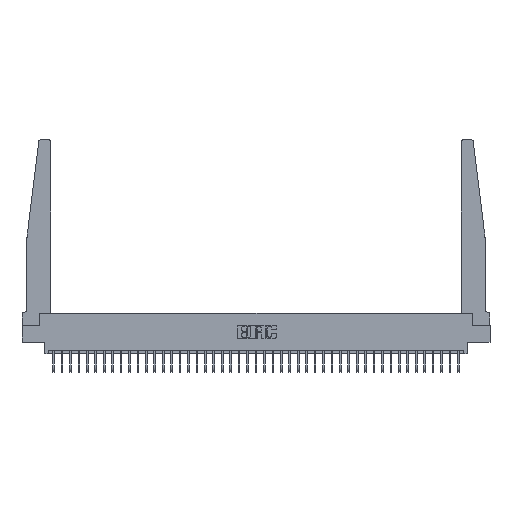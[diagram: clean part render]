
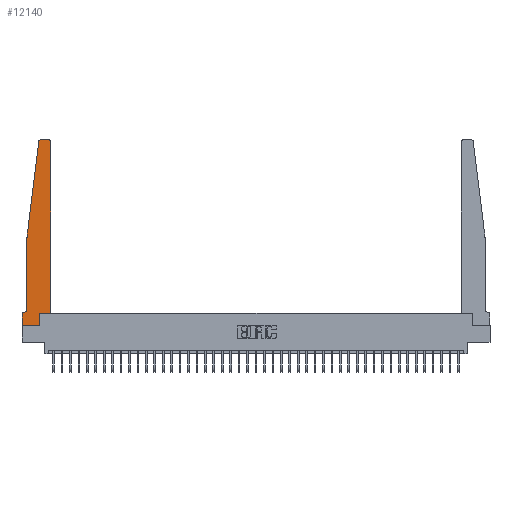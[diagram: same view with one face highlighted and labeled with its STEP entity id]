
A CAD part, top view. The second image highlights one B-rep face of the part: STEP entity #12140.
In plain terms, the highlighted planar face has unit normal (0, 0, 1).
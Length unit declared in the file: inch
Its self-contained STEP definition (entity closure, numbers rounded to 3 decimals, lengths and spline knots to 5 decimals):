
#183 = VECTOR ( 'NONE', #31343, 39.37008 ) ;
#203 = CARTESIAN_POINT ( 'NONE',  ( 0.065, 0.1875, 0.37 ) ) ;
#637 = LINE ( 'NONE', #17168, #20288 ) ;
#902 = EDGE_CURVE ( 'NONE', #23604, #21692, #637, .T. ) ;
#1043 = LINE ( 'NONE', #4830, #183 ) ;
#1441 = ORIENTED_EDGE ( 'NONE', *, *, #14153, .T. ) ;
#1564 = LINE ( 'NONE', #13579, #22797 ) ;
#2021 = ORIENTED_EDGE ( 'NONE', *, *, #902, .T. ) ;
#2184 = AXIS2_PLACEMENT_3D ( 'NONE', #25909, #10046, #28567 ) ;
#2865 = LINE ( 'NONE', #33511, #16244 ) ;
#3051 = ORIENTED_EDGE ( 'NONE', *, *, #7508, .T. ) ;
#3892 = DIRECTION ( 'NONE',  ( 1., 0., 0. ) ) ;
#4414 = VECTOR ( 'NONE', #10277, 39.37008 ) ;
#4465 = VERTEX_POINT ( 'NONE', #12247 ) ;
#4830 = CARTESIAN_POINT ( 'NONE',  ( 0., 0., 0.37 ) ) ;
#5205 = CARTESIAN_POINT ( 'NONE',  ( 0.425, 0.18, 0.37 ) ) ;
#5595 = CARTESIAN_POINT ( 'NONE',  ( 0.395, 2.75, 0.37 ) ) ;
#5954 = VECTOR ( 'NONE', #13725, 39.37008 ) ;
#7012 = DIRECTION ( 'NONE',  ( 0., -1., 0. ) ) ;
#7071 = DIRECTION ( 'NONE',  ( -0.122, -0.992, 0. ) ) ;
#7468 = CARTESIAN_POINT ( 'NONE',  ( 0.27653, 2.75, 0.37 ) ) ;
#7508 = EDGE_CURVE ( 'NONE', #26942, #15308, #1043, .T. ) ;
#8187 = PLANE ( 'NONE',  #27552 ) ;
#8340 = CARTESIAN_POINT ( 'NONE',  ( 0.2605, 0.18, 0.37 ) ) ;
#9812 = CARTESIAN_POINT ( 'NONE',  ( 0.015, 0.1875, 0.37 ) ) ;
#9906 = EDGE_CURVE ( 'NONE', #26784, #23604, #27130, .T. ) ;
#10035 = VECTOR ( 'NONE', #7071, 39.37008 ) ;
#10046 = DIRECTION ( 'NONE',  ( 0., 0., 1. ) ) ;
#10163 = ORIENTED_EDGE ( 'NONE', *, *, #12797, .T. ) ;
#10277 = DIRECTION ( 'NONE',  ( -1., 0., 0. ) ) ;
#10892 = CARTESIAN_POINT ( 'NONE',  ( 0., 0.1875, 0.37 ) ) ;
#11379 = AXIS2_PLACEMENT_3D ( 'NONE', #12219, #30676, #14899 ) ;
#11956 = EDGE_CURVE ( 'NONE', #15308, #26784, #26575, .T. ) ;
#12140 = ADVANCED_FACE ( 'NONE', ( #13755 ), #8187, .T. ) ;
#12219 = CARTESIAN_POINT ( 'NONE',  ( 0.395, 2.72, 0.37 ) ) ;
#12247 = CARTESIAN_POINT ( 'NONE',  ( 0.425, 2.72, 0.37 ) ) ;
#12759 = ORIENTED_EDGE ( 'NONE', *, *, #24546, .T. ) ;
#12797 = EDGE_CURVE ( 'NONE', #18553, #26942, #14105, .T. ) ;
#13114 = VERTEX_POINT ( 'NONE', #25265 ) ;
#13136 = EDGE_CURVE ( 'NONE', #4465, #14378, #32709, .T. ) ;
#13571 = DIRECTION ( 'NONE',  ( 0., 0., 1. ) ) ;
#13579 = CARTESIAN_POINT ( 'NONE',  ( 0.425, 0.18, 0.37 ) ) ;
#13725 = DIRECTION ( 'NONE',  ( 0., 1., 0. ) ) ;
#13755 = FACE_OUTER_BOUND ( 'NONE', #24244, .T. ) ;
#13914 = CARTESIAN_POINT ( 'NONE',  ( 0.015, 0.2375, 0.37 ) ) ;
#14105 = LINE ( 'NONE', #203, #28151 ) ;
#14153 = EDGE_CURVE ( 'NONE', #31173, #13114, #29361, .T. ) ;
#14378 = VERTEX_POINT ( 'NONE', #5595 ) ;
#14437 = CARTESIAN_POINT ( 'NONE',  ( 0.065, 1.25, 0.37 ) ) ;
#14899 = DIRECTION ( 'NONE',  ( 1., 0., 0. ) ) ;
#15308 = VERTEX_POINT ( 'NONE', #30436 ) ;
#15559 = CARTESIAN_POINT ( 'NONE',  ( 0., 0., 0.37 ) ) ;
#16200 = EDGE_CURVE ( 'NONE', #14378, #31173, #32601, .T. ) ;
#16244 = VECTOR ( 'NONE', #7012, 39.37008 ) ;
#16564 = DIRECTION ( 'NONE',  ( -1., 0., 0. ) ) ;
#16752 = VERTEX_POINT ( 'NONE', #26331 ) ;
#17168 = CARTESIAN_POINT ( 'NONE',  ( 0.425, 0.18, 0.37 ) ) ;
#18182 = DIRECTION ( 'NONE',  ( 1., 0., 0. ) ) ;
#18553 = VERTEX_POINT ( 'NONE', #9812 ) ;
#18780 = ORIENTED_EDGE ( 'NONE', *, *, #11956, .T. ) ;
#18931 = DIRECTION ( 'NONE',  ( -1., 0., 0. ) ) ;
#20288 = VECTOR ( 'NONE', #3892, 39.37008 ) ;
#20460 = CIRCLE ( 'NONE', #33569, 0.05 ) ;
#20798 = EDGE_CURVE ( 'NONE', #25878, #16752, #2865, .T. ) ;
#21692 = VERTEX_POINT ( 'NONE', #5205 ) ;
#22797 = VECTOR ( 'NONE', #32028, 39.37008 ) ;
#22939 = CARTESIAN_POINT ( 'NONE',  ( 0.065, 1.25, 0.37 ) ) ;
#23530 = ORIENTED_EDGE ( 'NONE', *, *, #30765, .T. ) ;
#23604 = VERTEX_POINT ( 'NONE', #29729 ) ;
#23612 = ORIENTED_EDGE ( 'NONE', *, *, #9906, .T. ) ;
#24244 = EDGE_LOOP ( 'NONE', ( #31942, #1441, #12759, #29942, #23530, #10163, #3051, #18780, #23612, #2021, #30874, #25366 ) ) ;
#24546 = EDGE_CURVE ( 'NONE', #13114, #25878, #24928, .T. ) ;
#24928 = LINE ( 'NONE', #22939, #10035 ) ;
#25257 = EDGE_CURVE ( 'NONE', #21692, #4465, #1564, .T. ) ;
#25265 = CARTESIAN_POINT ( 'NONE',  ( 0.24675, 2.72367, 0.37 ) ) ;
#25366 = ORIENTED_EDGE ( 'NONE', *, *, #13136, .T. ) ;
#25878 = VERTEX_POINT ( 'NONE', #14437 ) ;
#25909 = CARTESIAN_POINT ( 'NONE',  ( 0.27653, 2.72, 0.37 ) ) ;
#26129 = CARTESIAN_POINT ( 'NONE',  ( 0.25, 2.75, 0.37 ) ) ;
#26331 = CARTESIAN_POINT ( 'NONE',  ( 0.065, 0.2375, 0.37 ) ) ;
#26575 = LINE ( 'NONE', #15559, #32735 ) ;
#26784 = VERTEX_POINT ( 'NONE', #28805 ) ;
#26942 = VERTEX_POINT ( 'NONE', #10892 ) ;
#27130 = LINE ( 'NONE', #8340, #5954 ) ;
#27552 = AXIS2_PLACEMENT_3D ( 'NONE', #31910, #13571, #32022 ) ;
#28151 = VECTOR ( 'NONE', #18931, 39.37008 ) ;
#28567 = DIRECTION ( 'NONE',  ( 1., 0., 0. ) ) ;
#28805 = CARTESIAN_POINT ( 'NONE',  ( 0.2605, 0., 0.37 ) ) ;
#29361 = CIRCLE ( 'NONE', #2184, 0.03 ) ;
#29729 = CARTESIAN_POINT ( 'NONE',  ( 0.2605, 0.18, 0.37 ) ) ;
#29942 = ORIENTED_EDGE ( 'NONE', *, *, #20798, .T. ) ;
#30436 = CARTESIAN_POINT ( 'NONE',  ( 0., 0., 0.37 ) ) ;
#30676 = DIRECTION ( 'NONE',  ( 0., 0., 1. ) ) ;
#30765 = EDGE_CURVE ( 'NONE', #16752, #18553, #20460, .T. ) ;
#30874 = ORIENTED_EDGE ( 'NONE', *, *, #25257, .T. ) ;
#31173 = VERTEX_POINT ( 'NONE', #7468 ) ;
#31343 = DIRECTION ( 'NONE',  ( 0., -1., 0. ) ) ;
#31910 = CARTESIAN_POINT ( 'NONE',  ( 0., 0.1875, 0.37 ) ) ;
#31942 = ORIENTED_EDGE ( 'NONE', *, *, #16200, .T. ) ;
#32022 = DIRECTION ( 'NONE',  ( 1., 0., 0. ) ) ;
#32028 = DIRECTION ( 'NONE',  ( 0., 1., 0. ) ) ;
#32359 = DIRECTION ( 'NONE',  ( 0., 0., -1. ) ) ;
#32601 = LINE ( 'NONE', #26129, #4414 ) ;
#32709 = CIRCLE ( 'NONE', #11379, 0.03 ) ;
#32735 = VECTOR ( 'NONE', #18182, 39.37008 ) ;
#33511 = CARTESIAN_POINT ( 'NONE',  ( 0.065, 1.25, 0.37 ) ) ;
#33569 = AXIS2_PLACEMENT_3D ( 'NONE', #13914, #32359, #16564 ) ;
